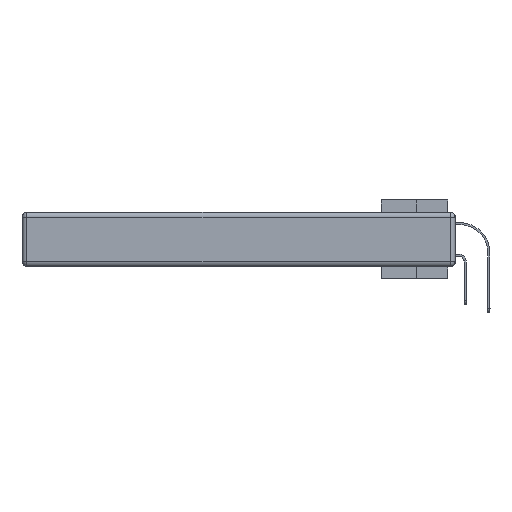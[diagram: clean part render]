
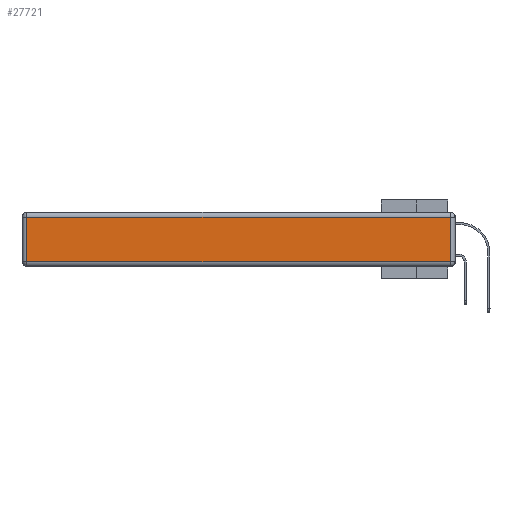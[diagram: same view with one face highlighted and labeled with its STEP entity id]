
A CAD part, left-side view. The second image highlights one B-rep face of the part: STEP entity #27721.
In plain terms, the highlighted planar face has unit normal (-1, 0, 0).
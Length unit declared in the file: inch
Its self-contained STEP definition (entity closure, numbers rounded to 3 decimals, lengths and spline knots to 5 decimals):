
#2925 = FACE_OUTER_BOUND ( 'NONE', #17973, .T. ) ;
#4443 = EDGE_CURVE ( 'NONE', #28734, #17407, #8067, .T. ) ;
#4639 = DIRECTION ( 'NONE',  ( 0., 0., -1. ) ) ;
#5085 = AXIS2_PLACEMENT_3D ( 'NONE', #9013, #30107, #5390 ) ;
#5390 = DIRECTION ( 'NONE',  ( 0., 0., 1. ) ) ;
#5774 = VECTOR ( 'NONE', #25848, 39.37008 ) ;
#8067 = LINE ( 'NONE', #26526, #9439 ) ;
#8167 = CARTESIAN_POINT ( 'NONE',  ( 0., 0., -0.313 ) ) ;
#9013 = CARTESIAN_POINT ( 'NONE',  ( 0., 0., -0.343 ) ) ;
#9151 = DIRECTION ( 'NONE',  ( 0., 1., 0. ) ) ;
#9439 = VECTOR ( 'NONE', #4639, 39.37008 ) ;
#10717 = ORIENTED_EDGE ( 'NONE', *, *, #29167, .T. ) ;
#11383 = EDGE_CURVE ( 'NONE', #17407, #17657, #13657, .T. ) ;
#13378 = CARTESIAN_POINT ( 'NONE',  ( 0., 0.03, -0.03 ) ) ;
#13466 = LINE ( 'NONE', #28697, #5774 ) ;
#13657 = LINE ( 'NONE', #8167, #21368 ) ;
#13847 = DIRECTION ( 'NONE',  ( 0., -1., 0. ) ) ;
#15804 = ORIENTED_EDGE ( 'NONE', *, *, #11383, .T. ) ;
#16220 = CARTESIAN_POINT ( 'NONE',  ( 0., 2.72, -0.313 ) ) ;
#16473 = EDGE_CURVE ( 'NONE', #17657, #22558, #13466, .T. ) ;
#17407 = VERTEX_POINT ( 'NONE', #16220 ) ;
#17657 = VERTEX_POINT ( 'NONE', #34440 ) ;
#17973 = EDGE_LOOP ( 'NONE', ( #15804, #20915, #10717, #26168 ) ) ;
#18452 = CARTESIAN_POINT ( 'NONE',  ( 0., 2.75, -0.03 ) ) ;
#18697 = CARTESIAN_POINT ( 'NONE',  ( 0., 2.72, -0.03 ) ) ;
#20915 = ORIENTED_EDGE ( 'NONE', *, *, #16473, .T. ) ;
#21368 = VECTOR ( 'NONE', #13847, 39.37008 ) ;
#22558 = VERTEX_POINT ( 'NONE', #13378 ) ;
#24166 = LINE ( 'NONE', #18452, #33005 ) ;
#25848 = DIRECTION ( 'NONE',  ( 0., 0., 1. ) ) ;
#26168 = ORIENTED_EDGE ( 'NONE', *, *, #4443, .T. ) ;
#26526 = CARTESIAN_POINT ( 'NONE',  ( 0., 2.72, -0.343 ) ) ;
#27721 = ADVANCED_FACE ( 'NONE', ( #2925 ), #30706, .T. ) ;
#28697 = CARTESIAN_POINT ( 'NONE',  ( 0., 0.03, -0.343 ) ) ;
#28734 = VERTEX_POINT ( 'NONE', #18697 ) ;
#29167 = EDGE_CURVE ( 'NONE', #22558, #28734, #24166, .T. ) ;
#30107 = DIRECTION ( 'NONE',  ( -1., 0., 0. ) ) ;
#30706 = PLANE ( 'NONE',  #5085 ) ;
#33005 = VECTOR ( 'NONE', #9151, 39.37008 ) ;
#34440 = CARTESIAN_POINT ( 'NONE',  ( 0., 0.03, -0.313 ) ) ;
